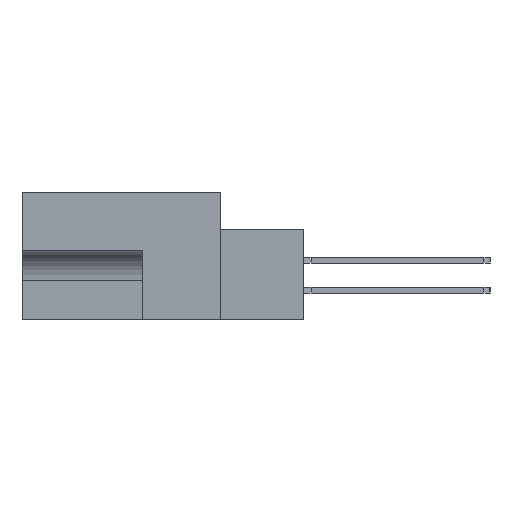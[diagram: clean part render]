
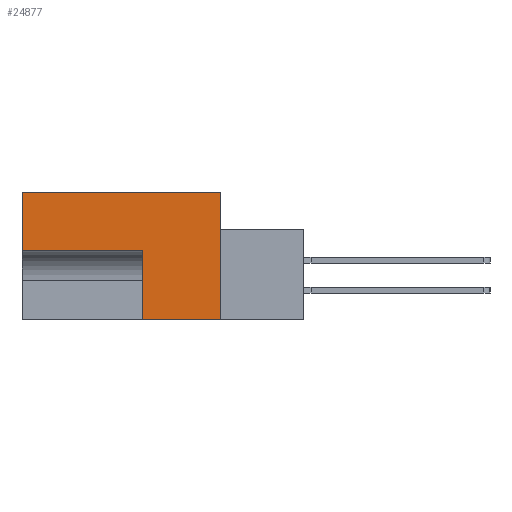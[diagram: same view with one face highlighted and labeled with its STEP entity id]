
A CAD part, left-side view. The second image highlights one B-rep face of the part: STEP entity #24877.
In plain terms, the highlighted planar face has unit normal (-1, 0, 0).
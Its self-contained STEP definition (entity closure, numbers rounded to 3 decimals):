
#2378 = DIRECTION ( 'NONE',  ( 0., 0., -1. ) ) ;
#2510 = CARTESIAN_POINT ( 'NONE',  ( 0., 0., 0. ) ) ;
#4020 = AXIS2_PLACEMENT_3D ( 'NONE', #20371, #30335, #39821 ) ;
#5589 = CARTESIAN_POINT ( 'NONE',  ( 0., 0., 0. ) ) ;
#5841 = LINE ( 'NONE', #2510, #9784 ) ;
#7646 = VERTEX_POINT ( 'NONE', #29983 ) ;
#8054 = EDGE_CURVE ( 'NONE', #27320, #7646, #30634, .T. ) ;
#8897 = ORIENTED_EDGE ( 'NONE', *, *, #31348, .F. ) ;
#9394 = EDGE_CURVE ( 'NONE', #22368, #27320, #5841, .T. ) ;
#9784 = VECTOR ( 'NONE', #2378, 1000. ) ;
#11707 = VERTEX_POINT ( 'NONE', #35573 ) ;
#11734 = EDGE_CURVE ( 'NONE', #21030, #22368, #21503, .T. ) ;
#12949 = ORIENTED_EDGE ( 'NONE', *, *, #14937, .F. ) ;
#13215 = LINE ( 'NONE', #33719, #16651 ) ;
#14841 = DIRECTION ( 'NONE',  ( 0., 0., 1. ) ) ;
#14853 = CARTESIAN_POINT ( 'NONE',  ( 0., 8.255, -6.172 ) ) ;
#14937 = EDGE_CURVE ( 'NONE', #7646, #29607, #26756, .T. ) ;
#16651 = VECTOR ( 'NONE', #14841, 1000. ) ;
#16934 = CARTESIAN_POINT ( 'NONE',  ( 0., 0., -13.487 ) ) ;
#17280 = DIRECTION ( 'NONE',  ( 0., 0., 1. ) ) ;
#19111 = LINE ( 'NONE', #21039, #29481 ) ;
#20371 = CARTESIAN_POINT ( 'NONE',  ( 0., 0., 0. ) ) ;
#21030 = VERTEX_POINT ( 'NONE', #25878 ) ;
#21039 = CARTESIAN_POINT ( 'NONE',  ( 0., 8.255, -6.172 ) ) ;
#21503 = LINE ( 'NONE', #32817, #26459 ) ;
#22368 = VERTEX_POINT ( 'NONE', #5589 ) ;
#23440 = EDGE_CURVE ( 'NONE', #29607, #11707, #19111, .T. ) ;
#23781 = DIRECTION ( 'NONE',  ( 0., 1., 0. ) ) ;
#24877 = ADVANCED_FACE ( 'NONE', ( #31248 ), #36121, .F. ) ;
#25243 = ORIENTED_EDGE ( 'NONE', *, *, #11734, .F. ) ;
#25878 = CARTESIAN_POINT ( 'NONE',  ( 0., 20.955, 0. ) ) ;
#26459 = VECTOR ( 'NONE', #29248, 1000. ) ;
#26756 = LINE ( 'NONE', #36040, #38092 ) ;
#27320 = VERTEX_POINT ( 'NONE', #16934 ) ;
#28167 = VECTOR ( 'NONE', #23781, 1000. ) ;
#29248 = DIRECTION ( 'NONE',  ( 0., -1., 0. ) ) ;
#29481 = VECTOR ( 'NONE', #39779, 1000. ) ;
#29607 = VERTEX_POINT ( 'NONE', #14853 ) ;
#29983 = CARTESIAN_POINT ( 'NONE',  ( 0., 8.255, -13.487 ) ) ;
#30335 = DIRECTION ( 'NONE',  ( 1., 0., 0. ) ) ;
#30634 = LINE ( 'NONE', #36190, #28167 ) ;
#31248 = FACE_OUTER_BOUND ( 'NONE', #39092, .T. ) ;
#31348 = EDGE_CURVE ( 'NONE', #11707, #21030, #13215, .T. ) ;
#32817 = CARTESIAN_POINT ( 'NONE',  ( 0., 11.506, 0. ) ) ;
#33719 = CARTESIAN_POINT ( 'NONE',  ( 0., 20.955, -13.487 ) ) ;
#35573 = CARTESIAN_POINT ( 'NONE',  ( 0., 20.955, -6.172 ) ) ;
#36040 = CARTESIAN_POINT ( 'NONE',  ( 0., 8.255, -13.487 ) ) ;
#36121 = PLANE ( 'NONE',  #4020 ) ;
#36190 = CARTESIAN_POINT ( 'NONE',  ( 0., -8.814, -13.487 ) ) ;
#36516 = ORIENTED_EDGE ( 'NONE', *, *, #23440, .F. ) ;
#37922 = ORIENTED_EDGE ( 'NONE', *, *, #9394, .F. ) ;
#38092 = VECTOR ( 'NONE', #17280, 1000. ) ;
#39092 = EDGE_LOOP ( 'NONE', ( #40366, #37922, #25243, #8897, #36516, #12949 ) ) ;
#39779 = DIRECTION ( 'NONE',  ( 0., 1., 0. ) ) ;
#39821 = DIRECTION ( 'NONE',  ( 0., 0., -1. ) ) ;
#40366 = ORIENTED_EDGE ( 'NONE', *, *, #8054, .F. ) ;
